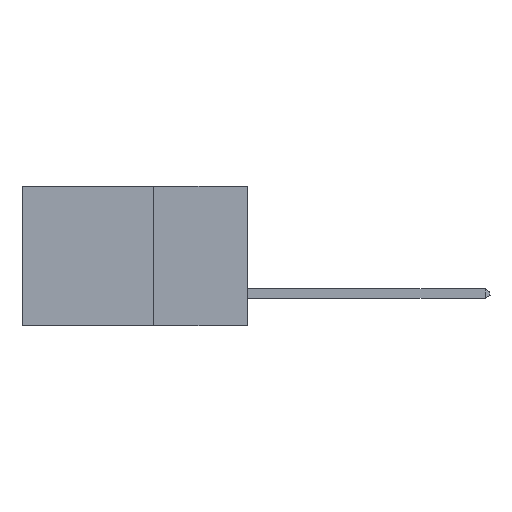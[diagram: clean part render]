
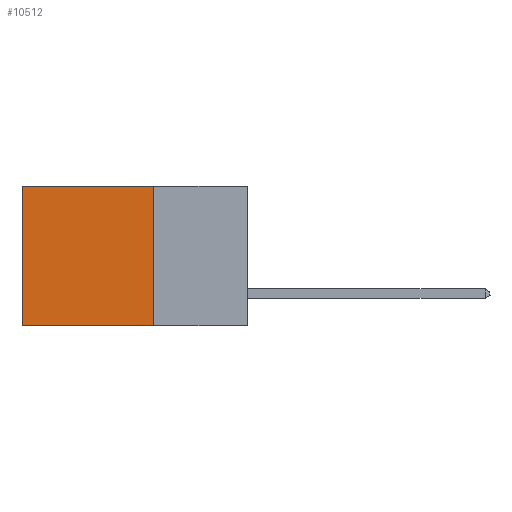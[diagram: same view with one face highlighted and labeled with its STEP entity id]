
A CAD part, left-side view. The second image highlights one B-rep face of the part: STEP entity #10512.
In plain terms, the highlighted planar face has unit normal (-1, 0, 0).
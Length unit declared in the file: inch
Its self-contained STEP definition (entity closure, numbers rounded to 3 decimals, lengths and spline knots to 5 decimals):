
#344 = ORIENTED_EDGE ( 'NONE', *, *, #1126, .F. ) ;
#379 = ORIENTED_EDGE ( 'NONE', *, *, #10724, .T. ) ;
#512 = DIRECTION ( 'NONE',  ( 0., 0., -1. ) ) ;
#696 = EDGE_LOOP ( 'NONE', ( #379, #12389, #344, #11927 ) ) ;
#872 = CARTESIAN_POINT ( 'NONE',  ( 0.298, 0.6, 0. ) ) ;
#1092 = LINE ( 'NONE', #1457, #10339 ) ;
#1126 = EDGE_CURVE ( 'NONE', #11186, #9905, #2640, .T. ) ;
#1457 = CARTESIAN_POINT ( 'NONE',  ( 0.298, 0.6, 0. ) ) ;
#1574 = CARTESIAN_POINT ( 'NONE',  ( 0.298, 0.25, 0. ) ) ;
#1978 = CARTESIAN_POINT ( 'NONE',  ( 0.298, 0.25, -0.37 ) ) ;
#1986 = VERTEX_POINT ( 'NONE', #11304 ) ;
#2640 = LINE ( 'NONE', #1574, #9740 ) ;
#2751 = VERTEX_POINT ( 'NONE', #872 ) ;
#2954 = CARTESIAN_POINT ( 'NONE',  ( 0.298, 0.25, 0. ) ) ;
#3255 = PLANE ( 'NONE',  #7496 ) ;
#3542 = DIRECTION ( 'NONE',  ( 0., 0., -1. ) ) ;
#3547 = VECTOR ( 'NONE', #10663, 39.37008 ) ;
#4139 = LINE ( 'NONE', #1978, #8947 ) ;
#6174 = LINE ( 'NONE', #2954, #3547 ) ;
#6280 = DIRECTION ( 'NONE',  ( 1., 0., 0. ) ) ;
#7496 = AXIS2_PLACEMENT_3D ( 'NONE', #8147, #6280, #11024 ) ;
#8045 = FACE_OUTER_BOUND ( 'NONE', #696, .T. ) ;
#8147 = CARTESIAN_POINT ( 'NONE',  ( 0.298, 0.25, 0. ) ) ;
#8947 = VECTOR ( 'NONE', #11861, 39.37008 ) ;
#9129 = CARTESIAN_POINT ( 'NONE',  ( 0.298, 0.25, 0. ) ) ;
#9740 = VECTOR ( 'NONE', #3542, 39.37008 ) ;
#9840 = CARTESIAN_POINT ( 'NONE',  ( 0.298, 0.25, -0.37 ) ) ;
#9905 = VERTEX_POINT ( 'NONE', #9840 ) ;
#10339 = VECTOR ( 'NONE', #512, 39.37008 ) ;
#10512 = ADVANCED_FACE ( 'NONE', ( #8045 ), #3255, .F. ) ;
#10663 = DIRECTION ( 'NONE',  ( 0., 1., 0. ) ) ;
#10724 = EDGE_CURVE ( 'NONE', #2751, #1986, #1092, .T. ) ;
#10933 = EDGE_CURVE ( 'NONE', #11186, #2751, #6174, .T. ) ;
#11024 = DIRECTION ( 'NONE',  ( 0., 0., -1. ) ) ;
#11186 = VERTEX_POINT ( 'NONE', #9129 ) ;
#11304 = CARTESIAN_POINT ( 'NONE',  ( 0.298, 0.6, -0.37 ) ) ;
#11861 = DIRECTION ( 'NONE',  ( 0., 1., 0. ) ) ;
#11927 = ORIENTED_EDGE ( 'NONE', *, *, #10933, .T. ) ;
#12185 = EDGE_CURVE ( 'NONE', #9905, #1986, #4139, .T. ) ;
#12389 = ORIENTED_EDGE ( 'NONE', *, *, #12185, .F. ) ;
